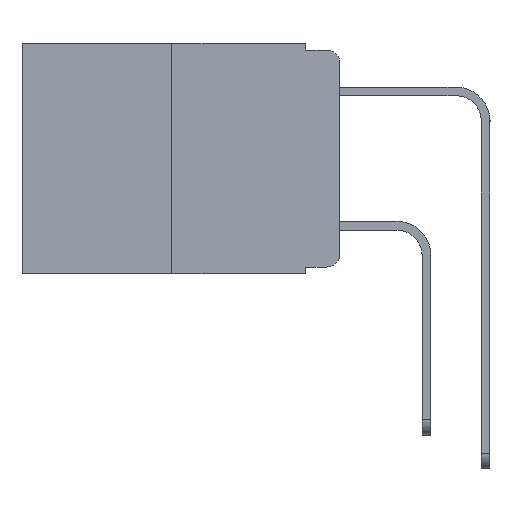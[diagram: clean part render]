
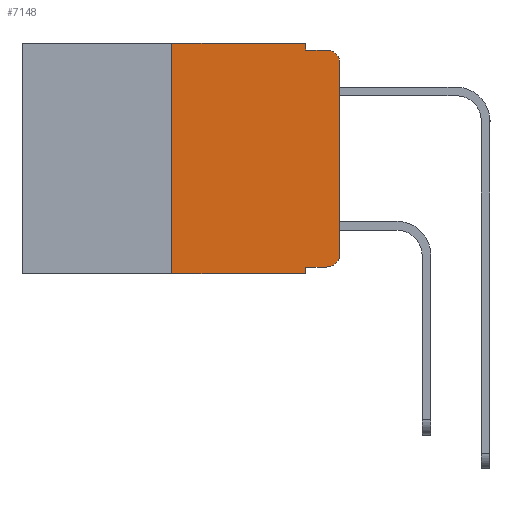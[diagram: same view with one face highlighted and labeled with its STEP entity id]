
A CAD part, left-side view. The second image highlights one B-rep face of the part: STEP entity #7148.
In plain terms, the highlighted planar face has unit normal (-1, 0, 0).
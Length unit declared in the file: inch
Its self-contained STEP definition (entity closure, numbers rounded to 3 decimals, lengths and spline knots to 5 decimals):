
#411 = CARTESIAN_POINT ( 'NONE',  ( 0., 0.02, -0.333 ) ) ;
#765 = CARTESIAN_POINT ( 'NONE',  ( 0., 0., -0.313 ) ) ;
#944 = LINE ( 'NONE', #1830, #5661 ) ;
#1113 = ORIENTED_EDGE ( 'NONE', *, *, #9041, .F. ) ;
#1315 = CARTESIAN_POINT ( 'NONE',  ( 0., 0.25, 0. ) ) ;
#1830 = CARTESIAN_POINT ( 'NONE',  ( 0., 0.051, -0.333 ) ) ;
#1870 = VECTOR ( 'NONE', #21840, 39.37008 ) ;
#2152 = VERTEX_POINT ( 'NONE', #411 ) ;
#2560 = AXIS2_PLACEMENT_3D ( 'NONE', #8195, #22202, #10196 ) ;
#2693 = DIRECTION ( 'NONE',  ( -1., 0., 0. ) ) ;
#2746 = DIRECTION ( 'NONE',  ( 0., -1., 0. ) ) ;
#3002 = PLANE ( 'NONE',  #3954 ) ;
#3050 = CARTESIAN_POINT ( 'NONE',  ( 0., 0., 0. ) ) ;
#3638 = ORIENTED_EDGE ( 'NONE', *, *, #21348, .F. ) ;
#3756 = EDGE_CURVE ( 'NONE', #8499, #2152, #944, .T. ) ;
#3954 = AXIS2_PLACEMENT_3D ( 'NONE', #22872, #16913, #5014 ) ;
#3995 = DIRECTION ( 'NONE',  ( 0., 0., 1. ) ) ;
#4195 = ORIENTED_EDGE ( 'NONE', *, *, #15741, .T. ) ;
#4474 = LINE ( 'NONE', #25421, #15036 ) ;
#4530 = VERTEX_POINT ( 'NONE', #20181 ) ;
#5014 = DIRECTION ( 'NONE',  ( 0., 0., -1. ) ) ;
#5137 = ORIENTED_EDGE ( 'NONE', *, *, #11734, .F. ) ;
#5551 = ORIENTED_EDGE ( 'NONE', *, *, #3756, .T. ) ;
#5661 = VECTOR ( 'NONE', #13719, 39.37008 ) ;
#5807 = LINE ( 'NONE', #22974, #9799 ) ;
#6366 = ORIENTED_EDGE ( 'NONE', *, *, #19774, .T. ) ;
#6424 = EDGE_CURVE ( 'NONE', #8499, #23635, #7181, .T. ) ;
#7084 = EDGE_CURVE ( 'NONE', #23468, #23635, #15538, .T. ) ;
#7148 = ADVANCED_FACE ( 'NONE', ( #13013 ), #3002, .F. ) ;
#7178 = VERTEX_POINT ( 'NONE', #12974 ) ;
#7181 = LINE ( 'NONE', #20566, #10599 ) ;
#7699 = VERTEX_POINT ( 'NONE', #12599 ) ;
#7719 = VERTEX_POINT ( 'NONE', #765 ) ;
#7992 = ORIENTED_EDGE ( 'NONE', *, *, #7084, .T. ) ;
#8195 = CARTESIAN_POINT ( 'NONE',  ( 0., 0.02, -0.03 ) ) ;
#8302 = CIRCLE ( 'NONE', #2560, 0.02 ) ;
#8499 = VERTEX_POINT ( 'NONE', #11381 ) ;
#8998 = LINE ( 'NONE', #23704, #1870 ) ;
#9041 = EDGE_CURVE ( 'NONE', #23468, #12268, #5807, .T. ) ;
#9335 = AXIS2_PLACEMENT_3D ( 'NONE', #14596, #2693, #16596 ) ;
#9799 = VECTOR ( 'NONE', #17011, 39.37008 ) ;
#10196 = DIRECTION ( 'NONE',  ( 0., 0., -1. ) ) ;
#10599 = VECTOR ( 'NONE', #22570, 39.37008 ) ;
#11146 = VECTOR ( 'NONE', #3995, 39.37008 ) ;
#11381 = CARTESIAN_POINT ( 'NONE',  ( 0., 0.051, -0.333 ) ) ;
#11734 = EDGE_CURVE ( 'NONE', #17037, #7699, #4474, .T. ) ;
#11928 = LINE ( 'NONE', #17590, #21967 ) ;
#12268 = VERTEX_POINT ( 'NONE', #1315 ) ;
#12599 = CARTESIAN_POINT ( 'NONE',  ( 0., 0.051, -0.01 ) ) ;
#12974 = CARTESIAN_POINT ( 'NONE',  ( 0., 0., -0.03 ) ) ;
#13013 = FACE_OUTER_BOUND ( 'NONE', #22882, .T. ) ;
#13505 = DIRECTION ( 'NONE',  ( 0., 0., -1. ) ) ;
#13633 = CARTESIAN_POINT ( 'NONE',  ( 0., 0.25, -0.343 ) ) ;
#13719 = DIRECTION ( 'NONE',  ( 0., -1., 0. ) ) ;
#14393 = EDGE_CURVE ( 'NONE', #7699, #4530, #8998, .T. ) ;
#14596 = CARTESIAN_POINT ( 'NONE',  ( 0., 0.02, -0.313 ) ) ;
#14917 = VECTOR ( 'NONE', #2746, 39.37008 ) ;
#15036 = VECTOR ( 'NONE', #13505, 39.37008 ) ;
#15538 = LINE ( 'NONE', #18575, #14917 ) ;
#15741 = EDGE_CURVE ( 'NONE', #7178, #4530, #8302, .T. ) ;
#16432 = LINE ( 'NONE', #3050, #11146 ) ;
#16596 = DIRECTION ( 'NONE',  ( 0., 0., -1. ) ) ;
#16913 = DIRECTION ( 'NONE',  ( 1., 0., 0. ) ) ;
#17011 = DIRECTION ( 'NONE',  ( 0., 0., 1. ) ) ;
#17037 = VERTEX_POINT ( 'NONE', #20715 ) ;
#17590 = CARTESIAN_POINT ( 'NONE',  ( 0., 0.473, 0. ) ) ;
#18144 = ORIENTED_EDGE ( 'NONE', *, *, #25546, .T. ) ;
#18575 = CARTESIAN_POINT ( 'NONE',  ( 0., 0.473, -0.343 ) ) ;
#19774 = EDGE_CURVE ( 'NONE', #7719, #7178, #16432, .T. ) ;
#20181 = CARTESIAN_POINT ( 'NONE',  ( 0., 0.02, -0.01 ) ) ;
#20303 = CARTESIAN_POINT ( 'NONE',  ( 0., 0.051, -0.343 ) ) ;
#20566 = CARTESIAN_POINT ( 'NONE',  ( 0., 0.051, 0. ) ) ;
#20715 = CARTESIAN_POINT ( 'NONE',  ( 0., 0.051, 0. ) ) ;
#21348 = EDGE_CURVE ( 'NONE', #12268, #17037, #11928, .T. ) ;
#21840 = DIRECTION ( 'NONE',  ( 0., -1., 0. ) ) ;
#21967 = VECTOR ( 'NONE', #25387, 39.37008 ) ;
#22202 = DIRECTION ( 'NONE',  ( -1., 0., 0. ) ) ;
#22400 = ORIENTED_EDGE ( 'NONE', *, *, #6424, .F. ) ;
#22570 = DIRECTION ( 'NONE',  ( 0., 0., -1. ) ) ;
#22872 = CARTESIAN_POINT ( 'NONE',  ( 0., 0.473, 0. ) ) ;
#22882 = EDGE_LOOP ( 'NONE', ( #6366, #4195, #23202, #5137, #3638, #1113, #7992, #22400, #5551, #18144 ) ) ;
#22974 = CARTESIAN_POINT ( 'NONE',  ( 0., 0.25, 0. ) ) ;
#23202 = ORIENTED_EDGE ( 'NONE', *, *, #14393, .F. ) ;
#23468 = VERTEX_POINT ( 'NONE', #13633 ) ;
#23635 = VERTEX_POINT ( 'NONE', #20303 ) ;
#23704 = CARTESIAN_POINT ( 'NONE',  ( 0., 0.051, -0.01 ) ) ;
#23824 = CIRCLE ( 'NONE', #9335, 0.02 ) ;
#25387 = DIRECTION ( 'NONE',  ( 0., -1., 0. ) ) ;
#25421 = CARTESIAN_POINT ( 'NONE',  ( 0., 0.051, 0. ) ) ;
#25546 = EDGE_CURVE ( 'NONE', #2152, #7719, #23824, .T. ) ;
